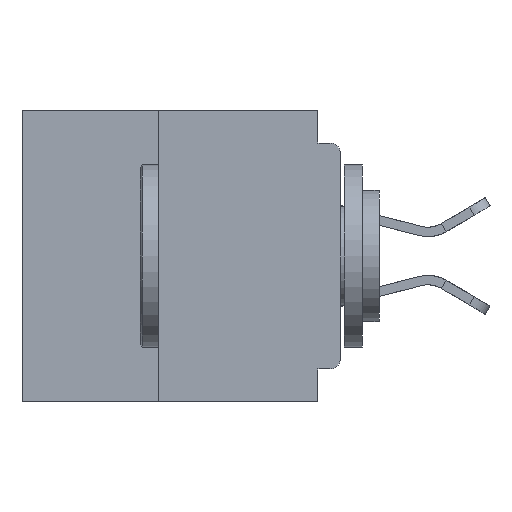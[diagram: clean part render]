
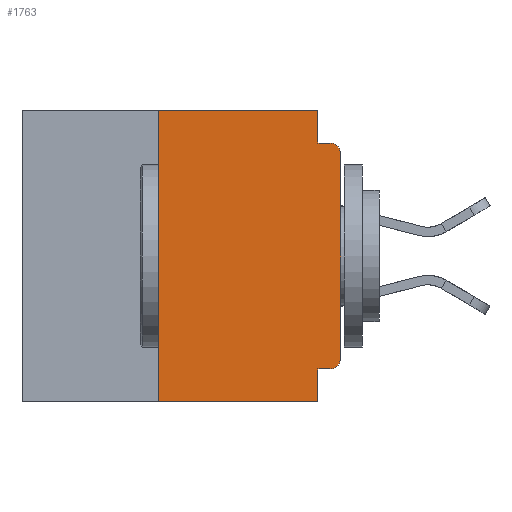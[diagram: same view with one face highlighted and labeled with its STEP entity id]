
A CAD part, left-side view. The second image highlights one B-rep face of the part: STEP entity #1763.
In plain terms, the highlighted planar face has unit normal (-1, 0, 0).
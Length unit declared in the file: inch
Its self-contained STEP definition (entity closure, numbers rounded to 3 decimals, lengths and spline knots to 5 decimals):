
#5 = CARTESIAN_POINT ( 'NONE',  ( 0., 0.015, -0.06 ) ) ;
#1088 = AXIS2_PLACEMENT_3D ( 'NONE', #5, #22542, #3255 ) ;
#1763 = ADVANCED_FACE ( 'NONE', ( #7624 ), #33779, .F. ) ;
#2018 = EDGE_CURVE ( 'NONE', #11755, #8687, #14681, .T. ) ;
#2481 = DIRECTION ( 'NONE',  ( -1., 0., 0. ) ) ;
#2643 = LINE ( 'NONE', #15349, #34866 ) ;
#2720 = ORIENTED_EDGE ( 'NONE', *, *, #12549, .F. ) ;
#3255 = DIRECTION ( 'NONE',  ( 0., 0., -1. ) ) ;
#3489 = CARTESIAN_POINT ( 'NONE',  ( 0., 0.25, -0.4 ) ) ;
#3644 = ORIENTED_EDGE ( 'NONE', *, *, #6529, .T. ) ;
#4453 = DIRECTION ( 'NONE',  ( 0., 0., -1. ) ) ;
#4714 = CIRCLE ( 'NONE', #9409, 0.015 ) ;
#4875 = VERTEX_POINT ( 'NONE', #30119 ) ;
#5021 = CARTESIAN_POINT ( 'NONE',  ( 0., 0., -0.355 ) ) ;
#5266 = VECTOR ( 'NONE', #21433, 39.37008 ) ;
#5338 = LINE ( 'NONE', #19985, #12912 ) ;
#5656 = EDGE_CURVE ( 'NONE', #27096, #4875, #41208, .T. ) ;
#5791 = ORIENTED_EDGE ( 'NONE', *, *, #2018, .F. ) ;
#6529 = EDGE_CURVE ( 'NONE', #4875, #8687, #26137, .T. ) ;
#6901 = CARTESIAN_POINT ( 'NONE',  ( 0., 0.031, -0.355 ) ) ;
#7115 = VECTOR ( 'NONE', #23984, 39.37008 ) ;
#7624 = FACE_OUTER_BOUND ( 'NONE', #7902, .T. ) ;
#7902 = EDGE_LOOP ( 'NONE', ( #22838, #3644, #5791, #31126, #10845, #21788, #25949, #2720, #33464, #25238 ) ) ;
#8687 = VERTEX_POINT ( 'NONE', #14660 ) ;
#9059 = AXIS2_PLACEMENT_3D ( 'NONE', #30593, #30442, #35071 ) ;
#9070 = CARTESIAN_POINT ( 'NONE',  ( 0., 0.031, 0. ) ) ;
#9409 = AXIS2_PLACEMENT_3D ( 'NONE', #21795, #2481, #24993 ) ;
#10845 = ORIENTED_EDGE ( 'NONE', *, *, #18784, .F. ) ;
#11755 = VERTEX_POINT ( 'NONE', #16374 ) ;
#11838 = VERTEX_POINT ( 'NONE', #13557 ) ;
#12549 = EDGE_CURVE ( 'NONE', #34951, #11838, #35513, .T. ) ;
#12638 = LINE ( 'NONE', #5021, #28692 ) ;
#12912 = VECTOR ( 'NONE', #29637, 39.37008 ) ;
#13317 = EDGE_CURVE ( 'NONE', #15871, #11838, #13879, .T. ) ;
#13557 = CARTESIAN_POINT ( 'NONE',  ( 0., 0.031, -0.4 ) ) ;
#13879 = LINE ( 'NONE', #18225, #5266 ) ;
#14080 = EDGE_CURVE ( 'NONE', #15871, #29745, #2643, .T. ) ;
#14506 = CARTESIAN_POINT ( 'NONE',  ( 0., 0., 0. ) ) ;
#14660 = CARTESIAN_POINT ( 'NONE',  ( 0., 0.015, -0.045 ) ) ;
#14681 = LINE ( 'NONE', #38538, #23157 ) ;
#15349 = CARTESIAN_POINT ( 'NONE',  ( 0., 0.25, -0.4 ) ) ;
#15871 = VERTEX_POINT ( 'NONE', #3489 ) ;
#16153 = EDGE_CURVE ( 'NONE', #21718, #34951, #12638, .T. ) ;
#16374 = CARTESIAN_POINT ( 'NONE',  ( 0., 0.031, -0.045 ) ) ;
#18225 = CARTESIAN_POINT ( 'NONE',  ( 0., 0.437, -0.4 ) ) ;
#18537 = EDGE_CURVE ( 'NONE', #32006, #11755, #5338, .T. ) ;
#18784 = EDGE_CURVE ( 'NONE', #29745, #32006, #28015, .T. ) ;
#19495 = VECTOR ( 'NONE', #33977, 39.37008 ) ;
#19985 = CARTESIAN_POINT ( 'NONE',  ( 0., 0.031, 0. ) ) ;
#21433 = DIRECTION ( 'NONE',  ( 0., -1., 0. ) ) ;
#21718 = VERTEX_POINT ( 'NONE', #36336 ) ;
#21788 = ORIENTED_EDGE ( 'NONE', *, *, #14080, .F. ) ;
#21790 = DIRECTION ( 'NONE',  ( 0., 0., 1. ) ) ;
#21795 = CARTESIAN_POINT ( 'NONE',  ( 0., 0.015, -0.34 ) ) ;
#22542 = DIRECTION ( 'NONE',  ( -1., 0., 0. ) ) ;
#22838 = ORIENTED_EDGE ( 'NONE', *, *, #5656, .T. ) ;
#23157 = VECTOR ( 'NONE', #36656, 39.37008 ) ;
#23984 = DIRECTION ( 'NONE',  ( 0., 0., 1. ) ) ;
#24833 = CARTESIAN_POINT ( 'NONE',  ( 0., 0., -0.34 ) ) ;
#24993 = DIRECTION ( 'NONE',  ( 0., 0., -1. ) ) ;
#25238 = ORIENTED_EDGE ( 'NONE', *, *, #35227, .T. ) ;
#25946 = VECTOR ( 'NONE', #4453, 39.37008 ) ;
#25949 = ORIENTED_EDGE ( 'NONE', *, *, #13317, .T. ) ;
#26137 = CIRCLE ( 'NONE', #1088, 0.015 ) ;
#27096 = VERTEX_POINT ( 'NONE', #24833 ) ;
#28015 = LINE ( 'NONE', #30617, #19495 ) ;
#28692 = VECTOR ( 'NONE', #40237, 39.37008 ) ;
#29637 = DIRECTION ( 'NONE',  ( 0., 0., -1. ) ) ;
#29745 = VERTEX_POINT ( 'NONE', #37867 ) ;
#30010 = CARTESIAN_POINT ( 'NONE',  ( 0., 0.031, -0.4 ) ) ;
#30119 = CARTESIAN_POINT ( 'NONE',  ( 0., 0., -0.06 ) ) ;
#30442 = DIRECTION ( 'NONE',  ( 1., 0., 0. ) ) ;
#30593 = CARTESIAN_POINT ( 'NONE',  ( 0., 0.437, 0. ) ) ;
#30617 = CARTESIAN_POINT ( 'NONE',  ( 0., 0.437, 0. ) ) ;
#31126 = ORIENTED_EDGE ( 'NONE', *, *, #18537, .F. ) ;
#32006 = VERTEX_POINT ( 'NONE', #9070 ) ;
#33464 = ORIENTED_EDGE ( 'NONE', *, *, #16153, .F. ) ;
#33779 = PLANE ( 'NONE',  #9059 ) ;
#33977 = DIRECTION ( 'NONE',  ( 0., -1., 0. ) ) ;
#34866 = VECTOR ( 'NONE', #21790, 39.37008 ) ;
#34951 = VERTEX_POINT ( 'NONE', #6901 ) ;
#35071 = DIRECTION ( 'NONE',  ( 0., 0., -1. ) ) ;
#35227 = EDGE_CURVE ( 'NONE', #21718, #27096, #4714, .T. ) ;
#35513 = LINE ( 'NONE', #30010, #25946 ) ;
#36336 = CARTESIAN_POINT ( 'NONE',  ( 0., 0.015, -0.355 ) ) ;
#36656 = DIRECTION ( 'NONE',  ( 0., -1., 0. ) ) ;
#37867 = CARTESIAN_POINT ( 'NONE',  ( 0., 0.25, 0. ) ) ;
#38538 = CARTESIAN_POINT ( 'NONE',  ( 0., 0., -0.045 ) ) ;
#40237 = DIRECTION ( 'NONE',  ( 0., 1., 0. ) ) ;
#41208 = LINE ( 'NONE', #14506, #7115 ) ;
